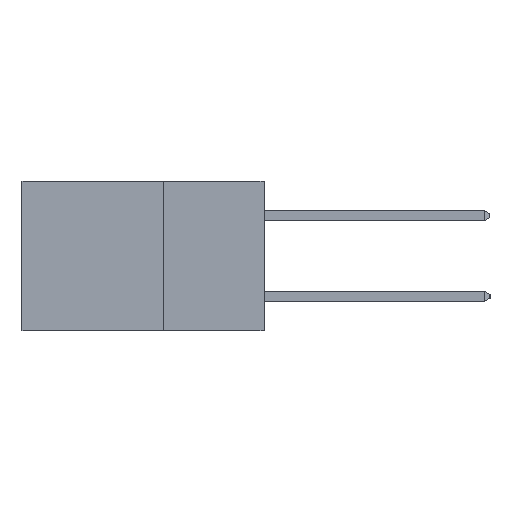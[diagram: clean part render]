
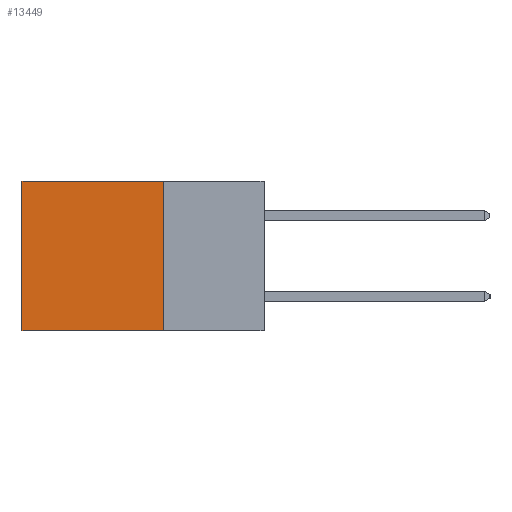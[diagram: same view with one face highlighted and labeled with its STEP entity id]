
A CAD part, left-side view. The second image highlights one B-rep face of the part: STEP entity #13449.
In plain terms, the highlighted planar face has unit normal (-1, 0, 0).
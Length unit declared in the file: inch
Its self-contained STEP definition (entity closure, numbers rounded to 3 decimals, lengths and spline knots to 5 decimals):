
#1203 = ORIENTED_EDGE ( 'NONE', *, *, #14297, .F. ) ;
#1280 = FACE_OUTER_BOUND ( 'NONE', #8945, .T. ) ;
#2137 = CARTESIAN_POINT ( 'NONE',  ( 0.2615, 0.25, 0. ) ) ;
#2338 = VECTOR ( 'NONE', #15912, 39.37008 ) ;
#2904 = LINE ( 'NONE', #3859, #6586 ) ;
#3297 = PLANE ( 'NONE',  #5177 ) ;
#3511 = VERTEX_POINT ( 'NONE', #17967 ) ;
#3859 = CARTESIAN_POINT ( 'NONE',  ( 0.2615, 0.25, -0.37 ) ) ;
#4282 = CARTESIAN_POINT ( 'NONE',  ( 0.2615, 0.6, -0.37 ) ) ;
#4884 = DIRECTION ( 'NONE',  ( 0., 0., -1. ) ) ;
#5177 = AXIS2_PLACEMENT_3D ( 'NONE', #12539, #14049, #4884 ) ;
#6586 = VECTOR ( 'NONE', #14577, 39.37008 ) ;
#6692 = LINE ( 'NONE', #8314, #14294 ) ;
#8314 = CARTESIAN_POINT ( 'NONE',  ( 0.2615, 0.25, -0.37 ) ) ;
#8588 = EDGE_CURVE ( 'NONE', #18139, #9192, #2904, .T. ) ;
#8739 = ORIENTED_EDGE ( 'NONE', *, *, #17162, .T. ) ;
#8945 = EDGE_LOOP ( 'NONE', ( #8739, #17149, #1203, #11358 ) ) ;
#9192 = VERTEX_POINT ( 'NONE', #12854 ) ;
#11028 = VERTEX_POINT ( 'NONE', #13921 ) ;
#11358 = ORIENTED_EDGE ( 'NONE', *, *, #19783, .T. ) ;
#12539 = CARTESIAN_POINT ( 'NONE',  ( 0.2615, 0.25, -0.37 ) ) ;
#12854 = CARTESIAN_POINT ( 'NONE',  ( 0.2615, 0.6, -0.37 ) ) ;
#12896 = DIRECTION ( 'NONE',  ( 0., 0., -1. ) ) ;
#13449 = ADVANCED_FACE ( 'NONE', ( #1280 ), #3297, .F. ) ;
#13531 = VECTOR ( 'NONE', #17983, 39.37008 ) ;
#13690 = CARTESIAN_POINT ( 'NONE',  ( 0.2615, 0.25, -0.37 ) ) ;
#13921 = CARTESIAN_POINT ( 'NONE',  ( 0.2615, 0.6, 0. ) ) ;
#14049 = DIRECTION ( 'NONE',  ( 1., 0., 0. ) ) ;
#14294 = VECTOR ( 'NONE', #12896, 39.37008 ) ;
#14297 = EDGE_CURVE ( 'NONE', #3511, #18139, #6692, .T. ) ;
#14574 = LINE ( 'NONE', #2137, #2338 ) ;
#14577 = DIRECTION ( 'NONE',  ( 0., 1., 0. ) ) ;
#15912 = DIRECTION ( 'NONE',  ( 0., 1., 0. ) ) ;
#17050 = LINE ( 'NONE', #4282, #13531 ) ;
#17149 = ORIENTED_EDGE ( 'NONE', *, *, #8588, .F. ) ;
#17162 = EDGE_CURVE ( 'NONE', #11028, #9192, #17050, .T. ) ;
#17967 = CARTESIAN_POINT ( 'NONE',  ( 0.2615, 0.25, 0. ) ) ;
#17983 = DIRECTION ( 'NONE',  ( 0., 0., -1. ) ) ;
#18139 = VERTEX_POINT ( 'NONE', #13690 ) ;
#19783 = EDGE_CURVE ( 'NONE', #3511, #11028, #14574, .T. ) ;
